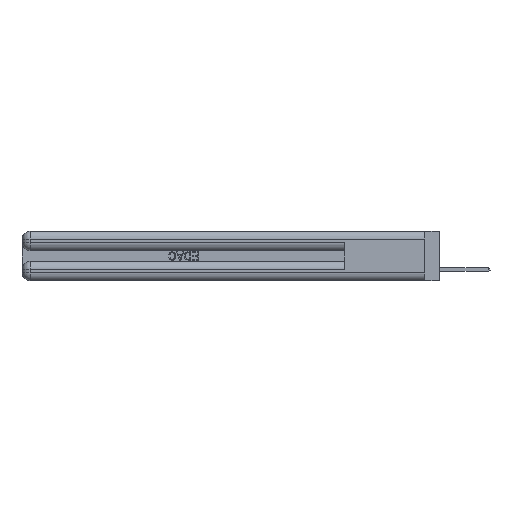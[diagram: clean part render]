
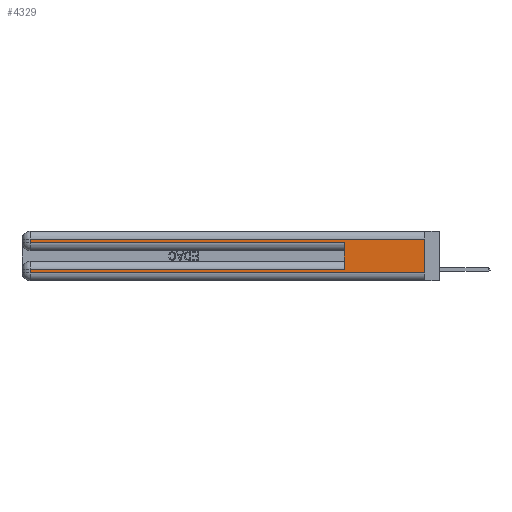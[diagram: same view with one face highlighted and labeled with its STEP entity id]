
A CAD part, left-side view. The second image highlights one B-rep face of the part: STEP entity #4329.
In plain terms, the highlighted planar face has unit normal (-1, 0, 0).
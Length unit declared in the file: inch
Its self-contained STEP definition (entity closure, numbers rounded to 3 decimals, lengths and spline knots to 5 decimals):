
#2625 = LINE ( 'NONE', #21387, #8139 ) ;
#2796 = DIRECTION ( 'NONE',  ( 0., 0., -1. ) ) ;
#3205 = CARTESIAN_POINT ( 'NONE',  ( 0., 0., 0.31 ) ) ;
#3643 = LINE ( 'NONE', #37715, #29511 ) ;
#4165 = VERTEX_POINT ( 'NONE', #29272 ) ;
#4329 = ADVANCED_FACE ( 'NONE', ( #14034 ), #20781, .F. ) ;
#5271 = ORIENTED_EDGE ( 'NONE', *, *, #31169, .T. ) ;
#5571 = ORIENTED_EDGE ( 'NONE', *, *, #14136, .T. ) ;
#5573 = VECTOR ( 'NONE', #37894, 39.37008 ) ;
#6472 = DIRECTION ( 'NONE',  ( 0., 0., -1. ) ) ;
#6476 = VERTEX_POINT ( 'NONE', #11062 ) ;
#7181 = CARTESIAN_POINT ( 'NONE',  ( 0., 0., 0.31 ) ) ;
#7604 = CARTESIAN_POINT ( 'NONE',  ( 0., 0., 0.06 ) ) ;
#8139 = VECTOR ( 'NONE', #14011, 39.37008 ) ;
#8864 = LINE ( 'NONE', #29389, #38608 ) ;
#9259 = DIRECTION ( 'NONE',  ( 0., -1., 0. ) ) ;
#10348 = CARTESIAN_POINT ( 'NONE',  ( 0., 2.94, 0.37 ) ) ;
#10682 = CARTESIAN_POINT ( 'NONE',  ( 0., 2.94, 0.31 ) ) ;
#11062 = CARTESIAN_POINT ( 'NONE',  ( 0., 2.94, 0.085 ) ) ;
#11361 = VERTEX_POINT ( 'NONE', #3205 ) ;
#12671 = EDGE_CURVE ( 'NONE', #15730, #17203, #8864, .T. ) ;
#13221 = DIRECTION ( 'NONE',  ( 1., 0., 0. ) ) ;
#14011 = DIRECTION ( 'NONE',  ( 0., 0., -1. ) ) ;
#14034 = FACE_OUTER_BOUND ( 'NONE', #36743, .T. ) ;
#14136 = EDGE_CURVE ( 'NONE', #11361, #27236, #26294, .T. ) ;
#15730 = VERTEX_POINT ( 'NONE', #29975 ) ;
#17203 = VERTEX_POINT ( 'NONE', #34652 ) ;
#20781 = PLANE ( 'NONE',  #22555 ) ;
#21387 = CARTESIAN_POINT ( 'NONE',  ( 0., 2.94, 0.37 ) ) ;
#22430 = DIRECTION ( 'NONE',  ( 0., -1., 0. ) ) ;
#22555 = AXIS2_PLACEMENT_3D ( 'NONE', #45244, #13221, #2796 ) ;
#23142 = DIRECTION ( 'NONE',  ( 0., 1., 0. ) ) ;
#23263 = LINE ( 'NONE', #37694, #28782 ) ;
#23473 = ORIENTED_EDGE ( 'NONE', *, *, #33142, .T. ) ;
#24942 = ORIENTED_EDGE ( 'NONE', *, *, #34817, .T. ) ;
#25650 = VECTOR ( 'NONE', #27243, 39.37008 ) ;
#26253 = ORIENTED_EDGE ( 'NONE', *, *, #12671, .T. ) ;
#26294 = LINE ( 'NONE', #7181, #28516 ) ;
#27054 = LINE ( 'NONE', #10348, #5573 ) ;
#27236 = VERTEX_POINT ( 'NONE', #10682 ) ;
#27243 = DIRECTION ( 'NONE',  ( 0., 0., 1. ) ) ;
#28174 = EDGE_CURVE ( 'NONE', #34150, #6476, #36136, .T. ) ;
#28516 = VECTOR ( 'NONE', #31803, 39.37008 ) ;
#28782 = VECTOR ( 'NONE', #6472, 39.37008 ) ;
#29272 = CARTESIAN_POINT ( 'NONE',  ( 0., 2.94, 0.06 ) ) ;
#29389 = CARTESIAN_POINT ( 'NONE',  ( 0., 0., 0.285 ) ) ;
#29511 = VECTOR ( 'NONE', #9259, 39.37008 ) ;
#29975 = CARTESIAN_POINT ( 'NONE',  ( 0., 2.94, 0.285 ) ) ;
#31169 = EDGE_CURVE ( 'NONE', #27236, #15730, #27054, .T. ) ;
#31257 = CARTESIAN_POINT ( 'NONE',  ( 0., 0.6, 0.145 ) ) ;
#31803 = DIRECTION ( 'NONE',  ( 0., 1., 0. ) ) ;
#32864 = ORIENTED_EDGE ( 'NONE', *, *, #40811, .F. ) ;
#33142 = EDGE_CURVE ( 'NONE', #6476, #4165, #2625, .T. ) ;
#33375 = LINE ( 'NONE', #31257, #25650 ) ;
#34150 = VERTEX_POINT ( 'NONE', #37318 ) ;
#34652 = CARTESIAN_POINT ( 'NONE',  ( 0., 0.6, 0.285 ) ) ;
#34817 = EDGE_CURVE ( 'NONE', #4165, #36214, #3643, .T. ) ;
#34906 = EDGE_CURVE ( 'NONE', #34150, #17203, #33375, .T. ) ;
#35669 = ORIENTED_EDGE ( 'NONE', *, *, #34906, .F. ) ;
#36136 = LINE ( 'NONE', #44405, #39416 ) ;
#36214 = VERTEX_POINT ( 'NONE', #7604 ) ;
#36743 = EDGE_LOOP ( 'NONE', ( #32864, #5571, #5271, #26253, #35669, #44699, #23473, #24942 ) ) ;
#37318 = CARTESIAN_POINT ( 'NONE',  ( 0., 0.6, 0.085 ) ) ;
#37694 = CARTESIAN_POINT ( 'NONE',  ( 0., 0., 0.37 ) ) ;
#37715 = CARTESIAN_POINT ( 'NONE',  ( 0., 0., 0.06 ) ) ;
#37894 = DIRECTION ( 'NONE',  ( 0., 0., -1. ) ) ;
#38608 = VECTOR ( 'NONE', #22430, 39.37008 ) ;
#39416 = VECTOR ( 'NONE', #23142, 39.37008 ) ;
#40811 = EDGE_CURVE ( 'NONE', #11361, #36214, #23263, .T. ) ;
#44405 = CARTESIAN_POINT ( 'NONE',  ( 0., 0., 0.085 ) ) ;
#44699 = ORIENTED_EDGE ( 'NONE', *, *, #28174, .T. ) ;
#45244 = CARTESIAN_POINT ( 'NONE',  ( 0., 0., 0.37 ) ) ;
